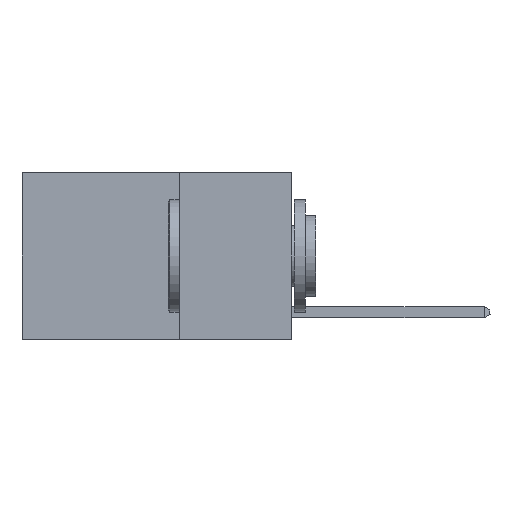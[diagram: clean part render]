
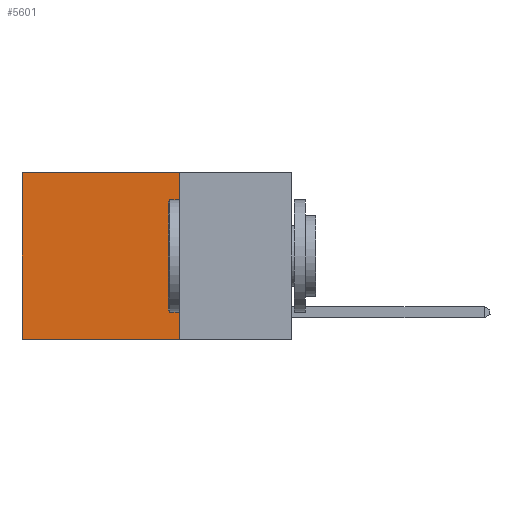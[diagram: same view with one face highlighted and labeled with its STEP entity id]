
A CAD part, left-side view. The second image highlights one B-rep face of the part: STEP entity #5601.
In plain terms, the highlighted planar face has unit normal (-1, 0, 0).
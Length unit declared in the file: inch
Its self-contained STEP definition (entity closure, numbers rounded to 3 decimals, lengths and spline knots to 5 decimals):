
#612 = ORIENTED_EDGE ( 'NONE', *, *, #1786, .F. ) ;
#1158 = CARTESIAN_POINT ( 'NONE',  ( 0.2625, 0.25, 0. ) ) ;
#1314 = VERTEX_POINT ( 'NONE', #8405 ) ;
#1786 = EDGE_CURVE ( 'NONE', #5687, #1314, #7092, .T. ) ;
#2473 = DIRECTION ( 'NONE',  ( 0., 1., 0. ) ) ;
#3173 = LINE ( 'NONE', #8143, #7503 ) ;
#3572 = DIRECTION ( 'NONE',  ( 0., 0., -1. ) ) ;
#3799 = FACE_OUTER_BOUND ( 'NONE', #14172, .T. ) ;
#4018 = EDGE_CURVE ( 'NONE', #5687, #11211, #13515, .T. ) ;
#4062 = CARTESIAN_POINT ( 'NONE',  ( 0.2625, 0.25, -0.37 ) ) ;
#4132 = DIRECTION ( 'NONE',  ( 0., 1., 0. ) ) ;
#5018 = EDGE_CURVE ( 'NONE', #11211, #13937, #3173, .T. ) ;
#5601 = ADVANCED_FACE ( 'NONE', ( #3799 ), #12332, .F. ) ;
#5687 = VERTEX_POINT ( 'NONE', #13933 ) ;
#6124 = ORIENTED_EDGE ( 'NONE', *, *, #5018, .T. ) ;
#6154 = ORIENTED_EDGE ( 'NONE', *, *, #4018, .T. ) ;
#7092 = LINE ( 'NONE', #10472, #10700 ) ;
#7320 = CARTESIAN_POINT ( 'NONE',  ( 0.2625, 0.25, 0. ) ) ;
#7426 = AXIS2_PLACEMENT_3D ( 'NONE', #7320, #9981, #15992 ) ;
#7503 = VECTOR ( 'NONE', #3572, 39.37008 ) ;
#7728 = EDGE_CURVE ( 'NONE', #1314, #13937, #8902, .T. ) ;
#8143 = CARTESIAN_POINT ( 'NONE',  ( 0.2625, 0.6, 0. ) ) ;
#8405 = CARTESIAN_POINT ( 'NONE',  ( 0.2625, 0.25, -0.37 ) ) ;
#8902 = LINE ( 'NONE', #4062, #11265 ) ;
#9774 = CARTESIAN_POINT ( 'NONE',  ( 0.2625, 0.6, 0. ) ) ;
#9981 = DIRECTION ( 'NONE',  ( 1., 0., 0. ) ) ;
#10472 = CARTESIAN_POINT ( 'NONE',  ( 0.2625, 0.25, 0. ) ) ;
#10700 = VECTOR ( 'NONE', #14202, 39.37008 ) ;
#10775 = VECTOR ( 'NONE', #2473, 39.37008 ) ;
#11211 = VERTEX_POINT ( 'NONE', #9774 ) ;
#11265 = VECTOR ( 'NONE', #4132, 39.37008 ) ;
#12072 = CARTESIAN_POINT ( 'NONE',  ( 0.2625, 0.6, -0.37 ) ) ;
#12332 = PLANE ( 'NONE',  #7426 ) ;
#13515 = LINE ( 'NONE', #1158, #10775 ) ;
#13933 = CARTESIAN_POINT ( 'NONE',  ( 0.2625, 0.25, 0. ) ) ;
#13937 = VERTEX_POINT ( 'NONE', #12072 ) ;
#14055 = ORIENTED_EDGE ( 'NONE', *, *, #7728, .F. ) ;
#14172 = EDGE_LOOP ( 'NONE', ( #6124, #14055, #612, #6154 ) ) ;
#14202 = DIRECTION ( 'NONE',  ( 0., 0., -1. ) ) ;
#15992 = DIRECTION ( 'NONE',  ( 0., 0., -1. ) ) ;
